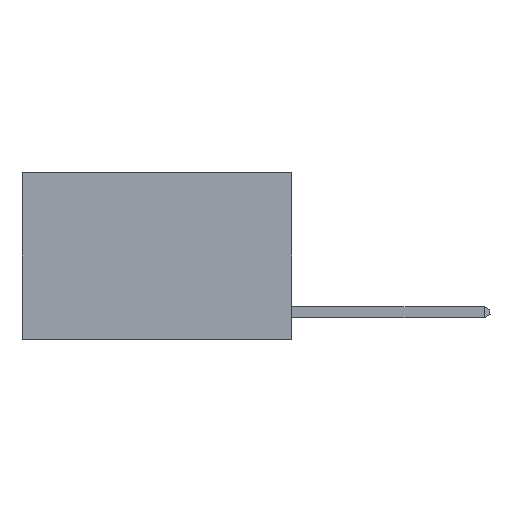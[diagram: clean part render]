
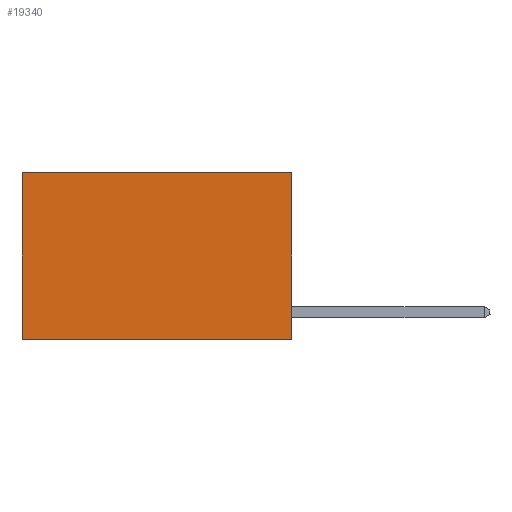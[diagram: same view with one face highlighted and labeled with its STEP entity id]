
A CAD part, left-side view. The second image highlights one B-rep face of the part: STEP entity #19340.
In plain terms, the highlighted planar face has unit normal (-1, 0, 0).
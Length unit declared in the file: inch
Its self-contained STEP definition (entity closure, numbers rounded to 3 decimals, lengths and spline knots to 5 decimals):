
#57 = VECTOR ( 'NONE', #11970, 39.37008 ) ;
#650 = DIRECTION ( 'NONE',  ( 1., 0., 0. ) ) ;
#770 = CARTESIAN_POINT ( 'NONE',  ( 0.2625, 0.6, 0. ) ) ;
#1078 = CARTESIAN_POINT ( 'NONE',  ( 0.2625, 0., 0. ) ) ;
#1571 = CARTESIAN_POINT ( 'NONE',  ( 0.2625, 0., 0. ) ) ;
#2386 = PLANE ( 'NONE',  #7622 ) ;
#2781 = CARTESIAN_POINT ( 'NONE',  ( 0.2625, 0.6, -0.37 ) ) ;
#3215 = LINE ( 'NONE', #1571, #8745 ) ;
#3599 = CARTESIAN_POINT ( 'NONE',  ( 0.2625, 0., 0. ) ) ;
#4668 = VERTEX_POINT ( 'NONE', #20134 ) ;
#5340 = LINE ( 'NONE', #8420, #57 ) ;
#5422 = ORIENTED_EDGE ( 'NONE', *, *, #13957, .T. ) ;
#6324 = ORIENTED_EDGE ( 'NONE', *, *, #9810, .T. ) ;
#7517 = VECTOR ( 'NONE', #15316, 39.37008 ) ;
#7622 = AXIS2_PLACEMENT_3D ( 'NONE', #1078, #650, #13784 ) ;
#8266 = VERTEX_POINT ( 'NONE', #3599 ) ;
#8420 = CARTESIAN_POINT ( 'NONE',  ( 0.2625, 0., -0.37 ) ) ;
#8745 = VECTOR ( 'NONE', #14828, 39.37008 ) ;
#9038 = LINE ( 'NONE', #770, #7517 ) ;
#9267 = VERTEX_POINT ( 'NONE', #2781 ) ;
#9810 = EDGE_CURVE ( 'NONE', #13516, #9267, #9038, .T. ) ;
#11294 = EDGE_LOOP ( 'NONE', ( #6324, #11644, #21265, #5422 ) ) ;
#11644 = ORIENTED_EDGE ( 'NONE', *, *, #17570, .F. ) ;
#11753 = CARTESIAN_POINT ( 'NONE',  ( 0.2625, 0.6, 0. ) ) ;
#11970 = DIRECTION ( 'NONE',  ( 0., 1., 0. ) ) ;
#12162 = FACE_OUTER_BOUND ( 'NONE', #11294, .T. ) ;
#12996 = CARTESIAN_POINT ( 'NONE',  ( 0.2625, 0., 0. ) ) ;
#13516 = VERTEX_POINT ( 'NONE', #11753 ) ;
#13784 = DIRECTION ( 'NONE',  ( 0., 0., -1. ) ) ;
#13957 = EDGE_CURVE ( 'NONE', #8266, #13516, #16236, .T. ) ;
#14828 = DIRECTION ( 'NONE',  ( 0., 0., -1. ) ) ;
#15316 = DIRECTION ( 'NONE',  ( 0., 0., -1. ) ) ;
#16236 = LINE ( 'NONE', #12996, #19416 ) ;
#16972 = EDGE_CURVE ( 'NONE', #8266, #4668, #3215, .T. ) ;
#17570 = EDGE_CURVE ( 'NONE', #4668, #9267, #5340, .T. ) ;
#19340 = ADVANCED_FACE ( 'NONE', ( #12162 ), #2386, .F. ) ;
#19416 = VECTOR ( 'NONE', #21228, 39.37008 ) ;
#20134 = CARTESIAN_POINT ( 'NONE',  ( 0.2625, 0., -0.37 ) ) ;
#21228 = DIRECTION ( 'NONE',  ( 0., 1., 0. ) ) ;
#21265 = ORIENTED_EDGE ( 'NONE', *, *, #16972, .F. ) ;
